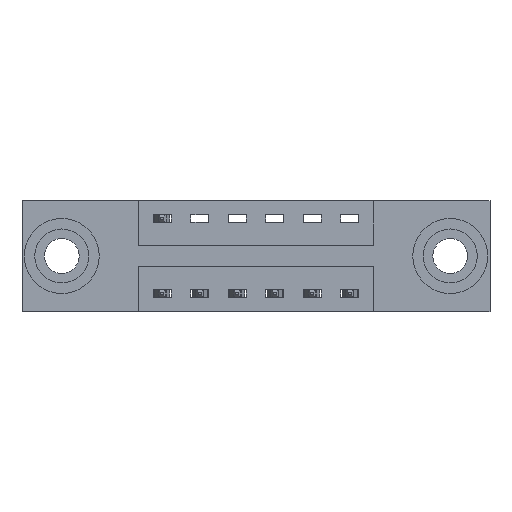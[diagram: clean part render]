
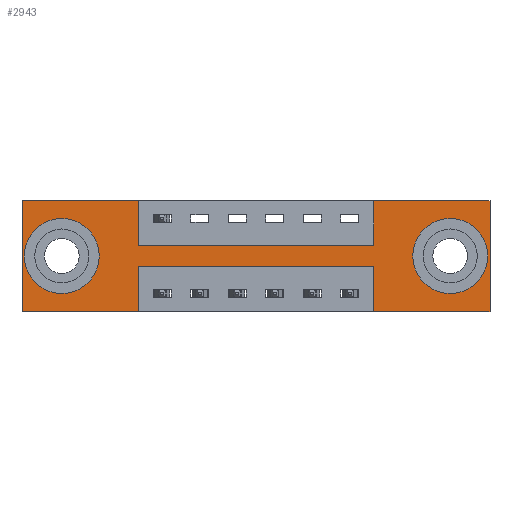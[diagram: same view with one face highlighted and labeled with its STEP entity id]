
A CAD part, front view. The second image highlights one B-rep face of the part: STEP entity #2943.
In plain terms, the highlighted planar face has unit normal (0, -1, 0).
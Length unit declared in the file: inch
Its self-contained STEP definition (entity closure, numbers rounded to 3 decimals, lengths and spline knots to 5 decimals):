
#49 = VECTOR ( 'NONE', #247, 39.37008 ) ;
#111 = ORIENTED_EDGE ( 'NONE', *, *, #2668, .T. ) ;
#219 = LINE ( 'NONE', #4690, #3672 ) ;
#247 = DIRECTION ( 'NONE',  ( -1., 0., 0. ) ) ;
#255 = EDGE_CURVE ( 'NONE', #7132, #5688, #219, .T. ) ;
#298 = ORIENTED_EDGE ( 'NONE', *, *, #8478, .T. ) ;
#302 = CARTESIAN_POINT ( 'NONE',  ( 0.3875, 0., 0. ) ) ;
#315 = EDGE_CURVE ( 'NONE', #2391, #3187, #7190, .T. ) ;
#445 = CARTESIAN_POINT ( 'NONE',  ( 0.3875, 0., -0.15 ) ) ;
#480 = CARTESIAN_POINT ( 'NONE',  ( 0.1325, 0., -0.185 ) ) ;
#804 = VERTEX_POINT ( 'NONE', #1246 ) ;
#916 = ORIENTED_EDGE ( 'NONE', *, *, #1698, .F. ) ;
#939 = ORIENTED_EDGE ( 'NONE', *, *, #1120, .F. ) ;
#942 = CARTESIAN_POINT ( 'NONE',  ( 0., 0., -0.37 ) ) ;
#950 = DIRECTION ( 'NONE',  ( 1., 0., 0. ) ) ;
#1049 = CIRCLE ( 'NONE', #7618, 0.078 ) ;
#1069 = CARTESIAN_POINT ( 'NONE',  ( 0.3875, 0., -0.15 ) ) ;
#1120 = EDGE_CURVE ( 'NONE', #4085, #1887, #2621, .T. ) ;
#1189 = EDGE_LOOP ( 'NONE', ( #4320, #5802 ) ) ;
#1229 = DIRECTION ( 'NONE',  ( 0., 0., 1. ) ) ;
#1246 = CARTESIAN_POINT ( 'NONE',  ( 0., 0., 0. ) ) ;
#1424 = CARTESIAN_POINT ( 'NONE',  ( 1.56, 0., -0.37 ) ) ;
#1520 = CARTESIAN_POINT ( 'NONE',  ( 0., 0., -0.37 ) ) ;
#1521 = CARTESIAN_POINT ( 'NONE',  ( 1.1725, 0., -0.37 ) ) ;
#1525 = DIRECTION ( 'NONE',  ( 0., 0., 1. ) ) ;
#1545 = DIRECTION ( 'NONE',  ( 0., 0., -1. ) ) ;
#1595 = ORIENTED_EDGE ( 'NONE', *, *, #5642, .F. ) ;
#1669 = CARTESIAN_POINT ( 'NONE',  ( 0., 0., 0. ) ) ;
#1698 = EDGE_CURVE ( 'NONE', #1887, #8253, #2268, .T. ) ;
#1774 = ORIENTED_EDGE ( 'NONE', *, *, #5918, .F. ) ;
#1887 = VERTEX_POINT ( 'NONE', #4547 ) ;
#1951 = VERTEX_POINT ( 'NONE', #3935 ) ;
#1987 = ORIENTED_EDGE ( 'NONE', *, *, #255, .F. ) ;
#1999 = CARTESIAN_POINT ( 'NONE',  ( 1.4275, 0., -0.263 ) ) ;
#2089 = DIRECTION ( 'NONE',  ( 0., 0., 1. ) ) ;
#2261 = CARTESIAN_POINT ( 'NONE',  ( 0.1325, 0., -0.185 ) ) ;
#2268 = LINE ( 'NONE', #8122, #7712 ) ;
#2360 = LINE ( 'NONE', #1669, #7805 ) ;
#2391 = VERTEX_POINT ( 'NONE', #7257 ) ;
#2486 = FACE_BOUND ( 'NONE', #7159, .T. ) ;
#2506 = EDGE_CURVE ( 'NONE', #8253, #5251, #8154, .T. ) ;
#2541 = CARTESIAN_POINT ( 'NONE',  ( 1.1725, 0., 0. ) ) ;
#2618 = CARTESIAN_POINT ( 'NONE',  ( 0., 0., 0. ) ) ;
#2621 = LINE ( 'NONE', #7337, #7842 ) ;
#2668 = EDGE_CURVE ( 'NONE', #5172, #5294, #6587, .T. ) ;
#2670 = DIRECTION ( 'NONE',  ( 1., 0., 0. ) ) ;
#2943 = ADVANCED_FACE ( 'NONE', ( #6246, #2486, #8042 ), #5147, .T. ) ;
#2996 = DIRECTION ( 'NONE',  ( 0., 0., 1. ) ) ;
#3027 = DIRECTION ( 'NONE',  ( 1., 0., 0. ) ) ;
#3028 = CARTESIAN_POINT ( 'NONE',  ( 1.4275, 0., -0.185 ) ) ;
#3072 = CARTESIAN_POINT ( 'NONE',  ( 1.4275, 0., -0.185 ) ) ;
#3184 = CARTESIAN_POINT ( 'NONE',  ( 0.1325, 0., -0.263 ) ) ;
#3187 = VERTEX_POINT ( 'NONE', #2541 ) ;
#3310 = LINE ( 'NONE', #8017, #8717 ) ;
#3373 = VECTOR ( 'NONE', #7577, 39.37008 ) ;
#3480 = CARTESIAN_POINT ( 'NONE',  ( 1.1725, 0., 0. ) ) ;
#3530 = ORIENTED_EDGE ( 'NONE', *, *, #4105, .F. ) ;
#3534 = ORIENTED_EDGE ( 'NONE', *, *, #315, .F. ) ;
#3574 = ORIENTED_EDGE ( 'NONE', *, *, #8818, .F. ) ;
#3672 = VECTOR ( 'NONE', #7023, 39.37008 ) ;
#3777 = DIRECTION ( 'NONE',  ( 0., 0., -1. ) ) ;
#3811 = DIRECTION ( 'NONE',  ( 0., 0., -1. ) ) ;
#3935 = CARTESIAN_POINT ( 'NONE',  ( 1.4275, 0., -0.107 ) ) ;
#4085 = VERTEX_POINT ( 'NONE', #4477 ) ;
#4105 = EDGE_CURVE ( 'NONE', #3187, #7132, #3310, .T. ) ;
#4190 = CARTESIAN_POINT ( 'NONE',  ( 0.3875, 0., -0.37 ) ) ;
#4320 = ORIENTED_EDGE ( 'NONE', *, *, #4600, .T. ) ;
#4477 = CARTESIAN_POINT ( 'NONE',  ( 1.1725, 0., -0.22 ) ) ;
#4547 = CARTESIAN_POINT ( 'NONE',  ( 0.3875, 0., -0.22 ) ) ;
#4600 = EDGE_CURVE ( 'NONE', #1951, #5026, #9161, .T. ) ;
#4690 = CARTESIAN_POINT ( 'NONE',  ( 1.56, 0., 0. ) ) ;
#4748 = LINE ( 'NONE', #6355, #8279 ) ;
#4757 = CIRCLE ( 'NONE', #5448, 0.078 ) ;
#4774 = VERTEX_POINT ( 'NONE', #302 ) ;
#4798 = VERTEX_POINT ( 'NONE', #1069 ) ;
#5026 = VERTEX_POINT ( 'NONE', #1999 ) ;
#5118 = VECTOR ( 'NONE', #1525, 39.37008 ) ;
#5135 = EDGE_CURVE ( 'NONE', #5026, #1951, #4757, .T. ) ;
#5147 = PLANE ( 'NONE',  #8710 ) ;
#5172 = VERTEX_POINT ( 'NONE', #5219 ) ;
#5219 = CARTESIAN_POINT ( 'NONE',  ( 0.1325, 0., -0.107 ) ) ;
#5251 = VERTEX_POINT ( 'NONE', #942 ) ;
#5294 = VERTEX_POINT ( 'NONE', #3184 ) ;
#5340 = DIRECTION ( 'NONE',  ( -1., 0., 0. ) ) ;
#5448 = AXIS2_PLACEMENT_3D ( 'NONE', #3028, #7984, #3777 ) ;
#5495 = LINE ( 'NONE', #2618, #3373 ) ;
#5539 = DIRECTION ( 'NONE',  ( 0., 1., 0. ) ) ;
#5609 = LINE ( 'NONE', #6008, #49 ) ;
#5642 = EDGE_CURVE ( 'NONE', #9103, #4085, #4748, .T. ) ;
#5688 = VERTEX_POINT ( 'NONE', #1424 ) ;
#5757 = VECTOR ( 'NONE', #2670, 39.37008 ) ;
#5802 = ORIENTED_EDGE ( 'NONE', *, *, #5135, .T. ) ;
#5813 = ORIENTED_EDGE ( 'NONE', *, *, #7584, .F. ) ;
#5821 = DIRECTION ( 'NONE',  ( 0., -1., 0. ) ) ;
#5918 = EDGE_CURVE ( 'NONE', #5688, #9103, #5609, .T. ) ;
#6008 = CARTESIAN_POINT ( 'NONE',  ( 0., 0., -0.37 ) ) ;
#6120 = VECTOR ( 'NONE', #7745, 39.37008 ) ;
#6246 = FACE_BOUND ( 'NONE', #1189, .T. ) ;
#6255 = VECTOR ( 'NONE', #5340, 39.37008 ) ;
#6317 = CARTESIAN_POINT ( 'NONE',  ( 0.3875, 0., 0. ) ) ;
#6355 = CARTESIAN_POINT ( 'NONE',  ( 1.1725, 0., -0.37 ) ) ;
#6578 = EDGE_CURVE ( 'NONE', #804, #4774, #2360, .T. ) ;
#6587 = CIRCLE ( 'NONE', #7958, 0.078 ) ;
#6714 = EDGE_CURVE ( 'NONE', #5251, #804, #5495, .T. ) ;
#6947 = ORIENTED_EDGE ( 'NONE', *, *, #6578, .F. ) ;
#7014 = DIRECTION ( 'NONE',  ( -1., 0., 0. ) ) ;
#7023 = DIRECTION ( 'NONE',  ( 0., 0., -1. ) ) ;
#7132 = VERTEX_POINT ( 'NONE', #8675 ) ;
#7159 = EDGE_LOOP ( 'NONE', ( #111, #298 ) ) ;
#7190 = LINE ( 'NONE', #3480, #5118 ) ;
#7227 = DIRECTION ( 'NONE',  ( 0., 1., 0. ) ) ;
#7257 = CARTESIAN_POINT ( 'NONE',  ( 1.1725, 0., -0.15 ) ) ;
#7337 = CARTESIAN_POINT ( 'NONE',  ( 0.3875, 0., -0.22 ) ) ;
#7402 = CARTESIAN_POINT ( 'NONE',  ( 0., 0., -0.37 ) ) ;
#7528 = ORIENTED_EDGE ( 'NONE', *, *, #6714, .F. ) ;
#7577 = DIRECTION ( 'NONE',  ( 0., 0., 1. ) ) ;
#7584 = EDGE_CURVE ( 'NONE', #4774, #4798, #8011, .T. ) ;
#7618 = AXIS2_PLACEMENT_3D ( 'NONE', #2261, #7227, #2996 ) ;
#7640 = LINE ( 'NONE', #445, #5757 ) ;
#7712 = VECTOR ( 'NONE', #8065, 39.37008 ) ;
#7745 = DIRECTION ( 'NONE',  ( 0., 0., -1. ) ) ;
#7805 = VECTOR ( 'NONE', #950, 39.37008 ) ;
#7842 = VECTOR ( 'NONE', #7014, 39.37008 ) ;
#7958 = AXIS2_PLACEMENT_3D ( 'NONE', #480, #5539, #1229 ) ;
#7984 = DIRECTION ( 'NONE',  ( 0., 1., 0. ) ) ;
#8011 = LINE ( 'NONE', #6317, #6120 ) ;
#8017 = CARTESIAN_POINT ( 'NONE',  ( 0., 0., 0. ) ) ;
#8023 = DIRECTION ( 'NONE',  ( 0., 1., 0. ) ) ;
#8042 = FACE_OUTER_BOUND ( 'NONE', #9048, .T. ) ;
#8065 = DIRECTION ( 'NONE',  ( 0., 0., -1. ) ) ;
#8070 = ORIENTED_EDGE ( 'NONE', *, *, #2506, .F. ) ;
#8122 = CARTESIAN_POINT ( 'NONE',  ( 0.3875, 0., -0.37 ) ) ;
#8154 = LINE ( 'NONE', #7402, #6255 ) ;
#8253 = VERTEX_POINT ( 'NONE', #4190 ) ;
#8279 = VECTOR ( 'NONE', #2089, 39.37008 ) ;
#8478 = EDGE_CURVE ( 'NONE', #5294, #5172, #1049, .T. ) ;
#8675 = CARTESIAN_POINT ( 'NONE',  ( 1.56, 0., 0. ) ) ;
#8710 = AXIS2_PLACEMENT_3D ( 'NONE', #1520, #5821, #1545 ) ;
#8717 = VECTOR ( 'NONE', #3027, 39.37008 ) ;
#8818 = EDGE_CURVE ( 'NONE', #4798, #2391, #7640, .T. ) ;
#9048 = EDGE_LOOP ( 'NONE', ( #916, #939, #1595, #1774, #1987, #3530, #3534, #3574, #5813, #6947, #7528, #8070 ) ) ;
#9087 = AXIS2_PLACEMENT_3D ( 'NONE', #3072, #8023, #3811 ) ;
#9103 = VERTEX_POINT ( 'NONE', #1521 ) ;
#9161 = CIRCLE ( 'NONE', #9087, 0.078 ) ;
